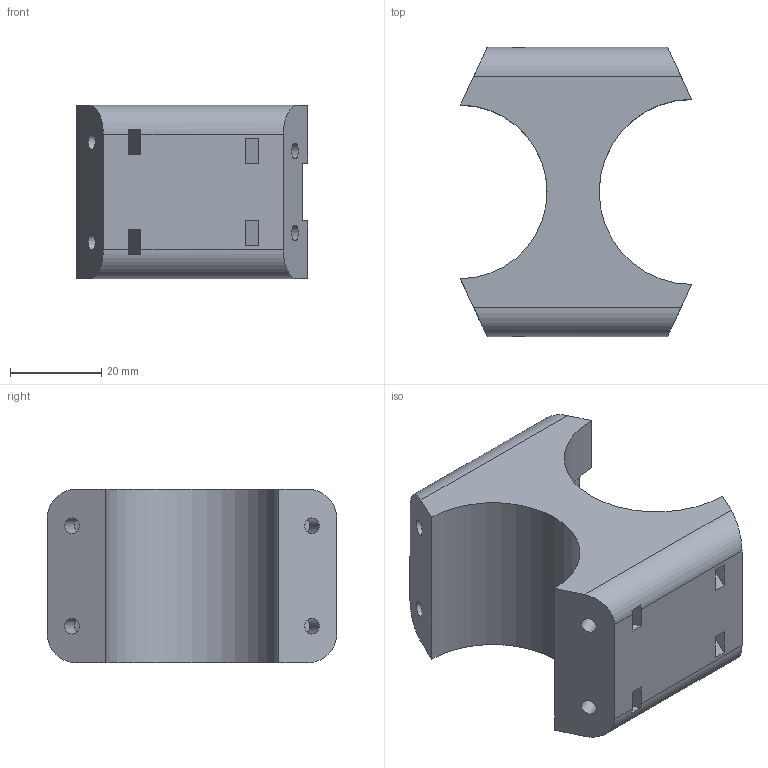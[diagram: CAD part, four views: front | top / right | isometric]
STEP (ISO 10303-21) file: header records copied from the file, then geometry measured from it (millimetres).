
FILE_DESCRIPTION (( 'STEP AP214' ), '1' );
FILE_NAME ('Trellais_Clamp_1.step', '2016-04-19T10:44:29', ( 'WarFairy' ), ( '' ), 'SwSTEP 2.0', 'SolidWorks 2015', '' );
FILE_SCHEMA (( 'AUTOMOTIVE_DESIGN' ));
Length unit declared in the file: millimetre
Products named in the file (1): Trellais_Clamp_1
Bounding box: 50.8 x 63.5 x 38.1 mm (x, y, z)
Volume: 65490.1 mm3; surface area: 15726.9 mm2
Topology: 1 solids, 1 shells, 90 faces, 228 edges, 152 vertices
Faces by surface type: plane 66, cylinder 24
Full cylindrical faces by diameter (mm): 3.5 x16
Entity records: 2678 total; most frequent: CARTESIAN_POINT 503, ORIENTED_EDGE 424, DIRECTION 418, EDGE_CURVE 212, LINE 156, VECTOR 156, VERTEX_POINT 152, EDGE_LOOP 134
